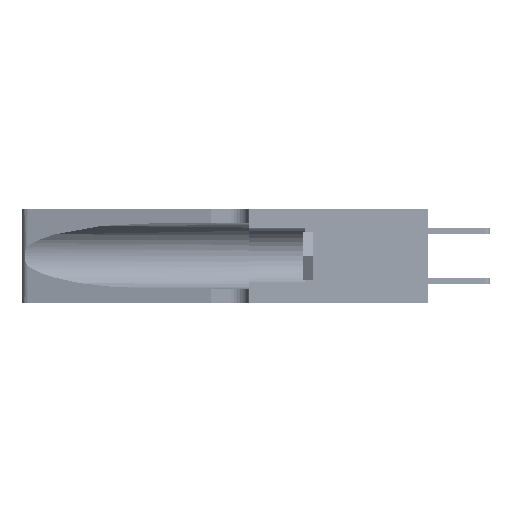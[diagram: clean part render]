
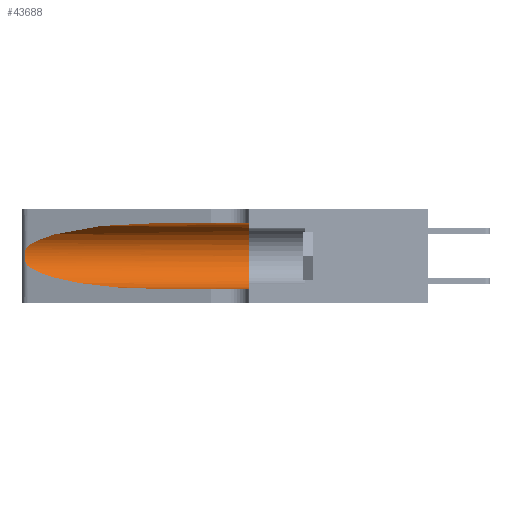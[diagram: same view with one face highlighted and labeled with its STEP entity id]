
A CAD part, left-side view. The second image highlights one B-rep face of the part: STEP entity #43688.
In plain terms, the highlighted cylindrical face has radius 3.308 mm (diameter 6.617 mm), a partial arc.
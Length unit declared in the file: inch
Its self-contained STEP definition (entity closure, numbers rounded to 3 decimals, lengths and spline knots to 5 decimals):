
#594 = ORIENTED_EDGE ( 'NONE', *, *, #17534, .T. ) ;
#643 = EDGE_CURVE ( 'NONE', #12151, #3562, #18973, .T. ) ;
#1529 = CARTESIAN_POINT ( 'NONE',  ( 0.26017, 1.23833, 0.17102 ) ) ;
#1919 = ORIENTED_EDGE ( 'NONE', *, *, #643, .T. ) ;
#2538 = VERTEX_POINT ( 'NONE', #36962 ) ;
#3562 = VERTEX_POINT ( 'NONE', #42862 ) ;
#3652 = VERTEX_POINT ( 'NONE', #17576 ) ;
#4325 = CARTESIAN_POINT ( 'NONE',  ( 0.25487, 1.22718, 0.14631 ) ) ;
#5034 = CARTESIAN_POINT ( 'NONE',  ( 0.25487, 1.22718, 0.14631 ) ) ;
#5345 = CARTESIAN_POINT ( 'NONE',  ( 0.25639, 1.23184, 0.21858 ) ) ;
#5483 = EDGE_LOOP ( 'NONE', ( #594, #48822, #1919, #16597, #36630, #37453 ) ) ;
#7876 = B_SPLINE_CURVE_WITH_KNOTS ( 'NONE', 3,
 ( #27759, #24082, #5345, #27927, #28582, #20416, #36323, #39983, #1529, #47669, #39651, #17045, #16691, #5034 ),
 .UNSPECIFIED., .F., .F.,
 ( 4, 2, 2, 2, 2, 2, 4 ),
 ( 0., 0.00027, 0.00053, 0.00107, 0.0016, 0.00187, 0.00214 ),
 .UNSPECIFIED. ) ;
#8912 = CARTESIAN_POINT ( 'NONE',  ( 0.18966, 0.96281, 0.31525 ) ) ;
#8994 = CARTESIAN_POINT ( 'NONE',  ( 0.1305, 0.72297, 0.05475 ) ) ;
#10165 = FACE_OUTER_BOUND ( 'NONE', #5483, .T. ) ;
#12151 = VERTEX_POINT ( 'NONE', #4325 ) ;
#13187 = CYLINDRICAL_SURFACE ( 'NONE', #24428, 0.13025 ) ;
#16544 = DIRECTION ( 'NONE',  ( 0., 0., 1. ) ) ;
#16597 = ORIENTED_EDGE ( 'NONE', *, *, #35126, .T. ) ;
#16691 = CARTESIAN_POINT ( 'NONE',  ( 0.25555, 1.22993, 0.14849 ) ) ;
#17045 = CARTESIAN_POINT ( 'NONE',  ( 0.25639, 1.23186, 0.15144 ) ) ;
#17534 = EDGE_CURVE ( 'NONE', #3652, #37716, #47151, .T. ) ;
#17576 = CARTESIAN_POINT ( 'NONE',  ( 0.1305, 0.72297, 0.31525 ) ) ;
#17947 = VECTOR ( 'NONE', #19289, 39.37008 ) ;
#18457 = DIRECTION ( 'NONE',  ( 0., -1., 0. ) ) ;
#18973 =( BOUNDED_CURVE ( )  B_SPLINE_CURVE ( 3, ( #47014, #43503, #31448, #8994 ),
 .UNSPECIFIED., .F., .F. ) 
 B_SPLINE_CURVE_WITH_KNOTS ( ( 4, 4 ),
 ( 3.44316, 4.71239 ),
 .UNSPECIFIED. ) 
 CURVE ( )  GEOMETRIC_REPRESENTATION_ITEM ( )  RATIONAL_B_SPLINE_CURVE ( ( 1., 0.87, 0.87, 1. ) ) 
 REPRESENTATION_ITEM ( '' )  );
#19289 = DIRECTION ( 'NONE',  ( 0., -1., 0. ) ) ;
#20416 = CARTESIAN_POINT ( 'NONE',  ( 0.26018, 1.23835, 0.19895 ) ) ;
#22338 = VECTOR ( 'NONE', #45002, 39.37008 ) ;
#24082 = CARTESIAN_POINT ( 'NONE',  ( 0.25555, 1.22994, 0.2215 ) ) ;
#24428 = AXIS2_PLACEMENT_3D ( 'NONE', #45716, #18457, #30311 ) ;
#25471 = AXIS2_PLACEMENT_3D ( 'NONE', #43010, #39352, #16544 ) ;
#26802 = CIRCLE ( 'NONE', #25471, 0.13025 ) ;
#27331 = CARTESIAN_POINT ( 'NONE',  ( 0.25487, 1.22718, 0.22369 ) ) ;
#27759 = CARTESIAN_POINT ( 'NONE',  ( 0.25487, 1.22718, 0.22369 ) ) ;
#27927 = CARTESIAN_POINT ( 'NONE',  ( 0.25787, 1.23484, 0.2124 ) ) ;
#28582 = CARTESIAN_POINT ( 'NONE',  ( 0.25854, 1.2359, 0.20912 ) ) ;
#29019 = CARTESIAN_POINT ( 'NONE',  ( 0.25487, 1.22718, 0.22369 ) ) ;
#29600 = CARTESIAN_POINT ( 'NONE',  ( 0.1305, 1.61858, 0.31525 ) ) ;
#30311 = DIRECTION ( 'NONE',  ( 0., 0., -1. ) ) ;
#30522 = LINE ( 'NONE', #34500, #17947 ) ;
#31448 = CARTESIAN_POINT ( 'NONE',  ( 0.18966, 0.96281, 0.05475 ) ) ;
#33499 = CARTESIAN_POINT ( 'NONE',  ( 0.1305, 0.35, 0.31525 ) ) ;
#33742 = EDGE_CURVE ( 'NONE', #3652, #38189, #43254, .T. ) ;
#34500 = CARTESIAN_POINT ( 'NONE',  ( 0.1305, 1.61858, 0.05475 ) ) ;
#35126 = EDGE_CURVE ( 'NONE', #3562, #2538, #30522, .T. ) ;
#36323 = CARTESIAN_POINT ( 'NONE',  ( 0.26075, 1.23896, 0.19203 ) ) ;
#36630 = ORIENTED_EDGE ( 'NONE', *, *, #45292, .F. ) ;
#36750 = CARTESIAN_POINT ( 'NONE',  ( 0.2373, 1.15595, 0.28018 ) ) ;
#36962 = CARTESIAN_POINT ( 'NONE',  ( 0.1305, 0.35, 0.05475 ) ) ;
#37453 = ORIENTED_EDGE ( 'NONE', *, *, #33742, .F. ) ;
#37716 = VERTEX_POINT ( 'NONE', #27331 ) ;
#38189 = VERTEX_POINT ( 'NONE', #33499 ) ;
#39352 = DIRECTION ( 'NONE',  ( 0., 1., 0. ) ) ;
#39651 = CARTESIAN_POINT ( 'NONE',  ( 0.25789, 1.23486, 0.15765 ) ) ;
#39983 = CARTESIAN_POINT ( 'NONE',  ( 0.26075, 1.23896, 0.178 ) ) ;
#42862 = CARTESIAN_POINT ( 'NONE',  ( 0.1305, 0.72297, 0.05475 ) ) ;
#43010 = CARTESIAN_POINT ( 'NONE',  ( 0.1305, 0.35, 0.185 ) ) ;
#43254 = LINE ( 'NONE', #29600, #22338 ) ;
#43503 = CARTESIAN_POINT ( 'NONE',  ( 0.2373, 1.15595, 0.08982 ) ) ;
#43688 = ADVANCED_FACE ( 'NONE', ( #10165 ), #13187, .F. ) ;
#45002 = DIRECTION ( 'NONE',  ( 0., -1., 0. ) ) ;
#45292 = EDGE_CURVE ( 'NONE', #38189, #2538, #26802, .T. ) ;
#45716 = CARTESIAN_POINT ( 'NONE',  ( 0.1305, 1.61858, 0.185 ) ) ;
#47014 = CARTESIAN_POINT ( 'NONE',  ( 0.25487, 1.22718, 0.14631 ) ) ;
#47100 = CARTESIAN_POINT ( 'NONE',  ( 0.1305, 0.72297, 0.31525 ) ) ;
#47151 =( BOUNDED_CURVE ( )  B_SPLINE_CURVE ( 3, ( #47100, #8912, #36750, #29019 ),
 .UNSPECIFIED., .F., .T. ) 
 B_SPLINE_CURVE_WITH_KNOTS ( ( 4, 4 ),
 ( 1.5708, 2.84003 ),
 .UNSPECIFIED. ) 
 CURVE ( )  GEOMETRIC_REPRESENTATION_ITEM ( )  RATIONAL_B_SPLINE_CURVE ( ( 1., 0.87, 0.87, 1. ) ) 
 REPRESENTATION_ITEM ( '' )  );
#47669 = CARTESIAN_POINT ( 'NONE',  ( 0.25856, 1.23593, 0.16098 ) ) ;
#48161 = EDGE_CURVE ( 'NONE', #37716, #12151, #7876, .T. ) ;
#48822 = ORIENTED_EDGE ( 'NONE', *, *, #48161, .T. ) ;
